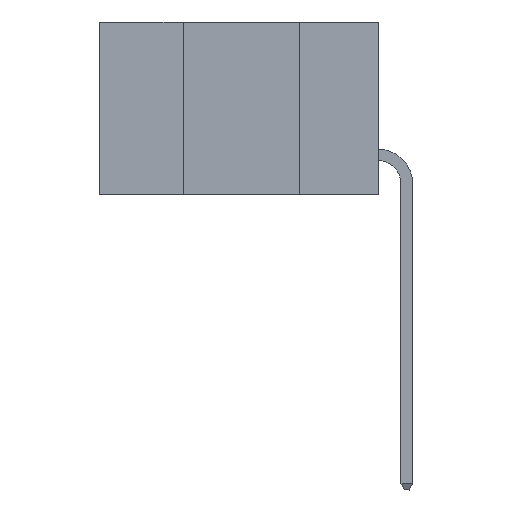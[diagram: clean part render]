
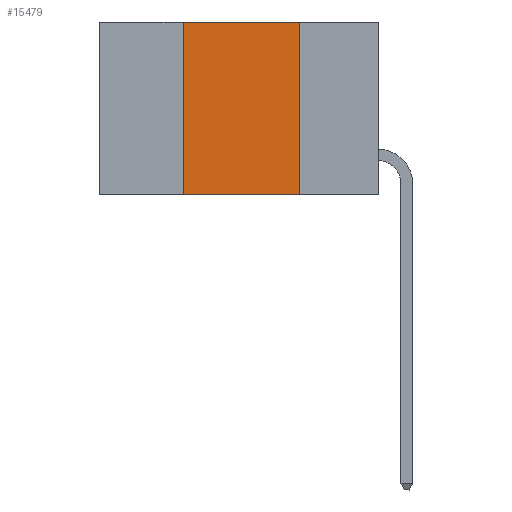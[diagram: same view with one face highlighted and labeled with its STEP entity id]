
A CAD part, left-side view. The second image highlights one B-rep face of the part: STEP entity #15479.
In plain terms, the highlighted planar face has unit normal (-1, 0, 0).
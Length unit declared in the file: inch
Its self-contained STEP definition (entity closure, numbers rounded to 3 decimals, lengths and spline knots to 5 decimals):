
#1422 = ORIENTED_EDGE ( 'NONE', *, *, #5927, .F. ) ;
#1578 = VECTOR ( 'NONE', #5316, 39.37008 ) ;
#2263 = CARTESIAN_POINT ( 'NONE',  ( 0., 0.6, 0. ) ) ;
#3000 = ORIENTED_EDGE ( 'NONE', *, *, #8940, .F. ) ;
#3274 = ORIENTED_EDGE ( 'NONE', *, *, #3447, .F. ) ;
#3447 = EDGE_CURVE ( 'NONE', #23167, #14440, #19262, .T. ) ;
#3538 = EDGE_LOOP ( 'NONE', ( #1422, #3274, #3000, #16772 ) ) ;
#4533 = VERTEX_POINT ( 'NONE', #8084 ) ;
#4643 = CARTESIAN_POINT ( 'NONE',  ( 0., 0.17, -0.37 ) ) ;
#5058 = LINE ( 'NONE', #10999, #12891 ) ;
#5172 = VECTOR ( 'NONE', #8457, 39.37008 ) ;
#5316 = DIRECTION ( 'NONE',  ( 0., -1., 0. ) ) ;
#5927 = EDGE_CURVE ( 'NONE', #14440, #4533, #18306, .T. ) ;
#6428 = VECTOR ( 'NONE', #10710, 39.37008 ) ;
#6471 = LINE ( 'NONE', #23446, #5172 ) ;
#7564 = DIRECTION ( 'NONE',  ( 1., 0., 0. ) ) ;
#8084 = CARTESIAN_POINT ( 'NONE',  ( 0., 0.17, -0.37 ) ) ;
#8457 = DIRECTION ( 'NONE',  ( 0., 0., 1. ) ) ;
#8940 = EDGE_CURVE ( 'NONE', #20380, #23167, #6471, .T. ) ;
#9156 = DIRECTION ( 'NONE',  ( 0., -1., 0. ) ) ;
#10710 = DIRECTION ( 'NONE',  ( 0., 0., -1. ) ) ;
#10999 = CARTESIAN_POINT ( 'NONE',  ( 0., 0.6, -0.37 ) ) ;
#11280 = FACE_OUTER_BOUND ( 'NONE', #3538, .T. ) ;
#11751 = CARTESIAN_POINT ( 'NONE',  ( 0., 0.42, -0.37 ) ) ;
#12891 = VECTOR ( 'NONE', #9156, 39.37008 ) ;
#14027 = EDGE_CURVE ( 'NONE', #20380, #4533, #5058, .T. ) ;
#14440 = VERTEX_POINT ( 'NONE', #18965 ) ;
#15479 = ADVANCED_FACE ( 'NONE', ( #11280 ), #20465, .F. ) ;
#15677 = AXIS2_PLACEMENT_3D ( 'NONE', #20584, #7564, #20349 ) ;
#16768 = CARTESIAN_POINT ( 'NONE',  ( 0., 0.42, 0. ) ) ;
#16772 = ORIENTED_EDGE ( 'NONE', *, *, #14027, .T. ) ;
#18306 = LINE ( 'NONE', #4643, #6428 ) ;
#18965 = CARTESIAN_POINT ( 'NONE',  ( 0., 0.17, 0. ) ) ;
#19262 = LINE ( 'NONE', #2263, #1578 ) ;
#20349 = DIRECTION ( 'NONE',  ( 0., 0., -1. ) ) ;
#20380 = VERTEX_POINT ( 'NONE', #11751 ) ;
#20465 = PLANE ( 'NONE',  #15677 ) ;
#20584 = CARTESIAN_POINT ( 'NONE',  ( 0., 0.6, 0. ) ) ;
#23167 = VERTEX_POINT ( 'NONE', #16768 ) ;
#23446 = CARTESIAN_POINT ( 'NONE',  ( 0., 0.42, -0.37 ) ) ;
